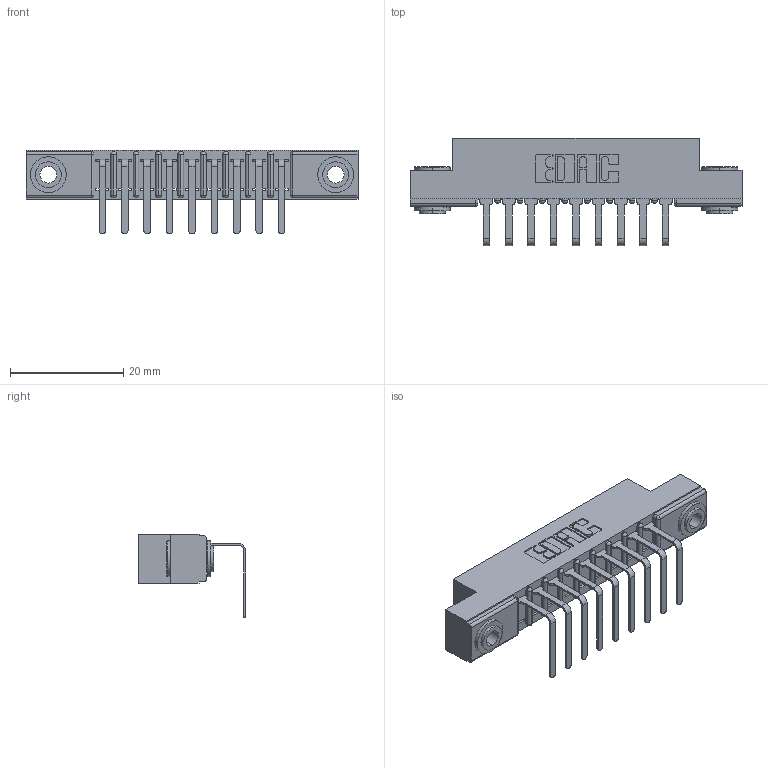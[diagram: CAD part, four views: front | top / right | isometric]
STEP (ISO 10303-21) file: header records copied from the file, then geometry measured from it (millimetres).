
FILE_DESCRIPTION (( 'STEP AP203' ), '1' );
FILE_NAME ('307-009-558-103.STEP', '2019-09-04T12:05:23', ( '' ), ( '' ), 'SwSTEP 2.0', 'SolidWorks 2016', '' );
FILE_SCHEMA (( 'CONFIG_CONTROL_DESIGN' ));
Length unit declared in the file: inch
Products named in the file (4): 307 Part_.156 Dia Mounting Holes; 307-009-558-103; 345-250-002_345-250-002-102; 307-290-001_558 - 2 (Single)
Assembly tree (12 placements, depth 2):
  307-009-558-103
    307 Part_.156 Dia Mounting Holes
    307-290-001_558 - 2 (Single)  x9
    345-250-002_345-250-002-102  x2
Bounding box: 58.67 x 18.96 x 14.81 mm (x, y, z)
Volume: 3778.9 mm3; surface area: 5869.8 mm2
Topology: 12 solids, 12 shells, 720 faces, 2001 edges, 1290 vertices
Faces by surface type: plane 445, cylinder 247, sphere 20, cone 8
Entity records: 12953 total; most frequent: CARTESIAN_POINT 2149, ORIENTED_EDGE 2126, DIRECTION 2125, EDGE_CURVE 1063, LINE 793, VECTOR 793, VERTEX_POINT 690, AXIS2_PLACEMENT_3D 666
